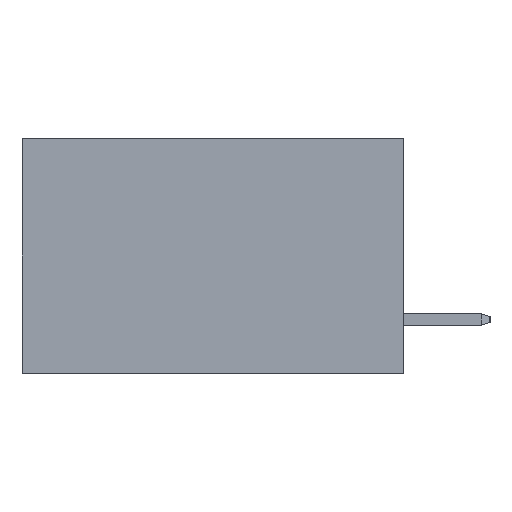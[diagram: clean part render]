
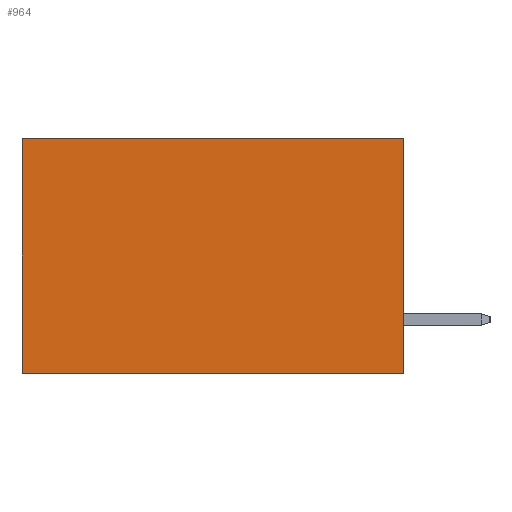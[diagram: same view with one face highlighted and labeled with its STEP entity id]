
A CAD part, left-side view. The second image highlights one B-rep face of the part: STEP entity #964.
In plain terms, the highlighted planar face has unit normal (-1, 0, 0).
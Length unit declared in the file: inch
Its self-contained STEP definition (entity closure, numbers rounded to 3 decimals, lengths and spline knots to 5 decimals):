
#555 = CARTESIAN_POINT ( 'NONE',  ( 0.2875, 0., 0. ) ) ;
#858 = CARTESIAN_POINT ( 'NONE',  ( 0.2875, 0., 0. ) ) ;
#964 = ADVANCED_FACE ( 'NONE', ( #3666 ), #6240, .F. ) ;
#1748 = VERTEX_POINT ( 'NONE', #2897 ) ;
#1966 = ORIENTED_EDGE ( 'NONE', *, *, #9739, .T. ) ;
#2611 = CARTESIAN_POINT ( 'NONE',  ( 0.2875, 0., 0. ) ) ;
#2897 = CARTESIAN_POINT ( 'NONE',  ( 0.2875, 0., -0.37 ) ) ;
#3125 = CARTESIAN_POINT ( 'NONE',  ( 0.2875, 0.6, 0. ) ) ;
#3482 = EDGE_CURVE ( 'NONE', #7500, #5282, #8560, .T. ) ;
#3639 = EDGE_CURVE ( 'NONE', #9727, #1748, #5838, .T. ) ;
#3666 = FACE_OUTER_BOUND ( 'NONE', #4972, .T. ) ;
#3714 = AXIS2_PLACEMENT_3D ( 'NONE', #555, #6927, #9453 ) ;
#4009 = EDGE_CURVE ( 'NONE', #1748, #5282, #5455, .T. ) ;
#4097 = DIRECTION ( 'NONE',  ( 0., 1., 0. ) ) ;
#4133 = CARTESIAN_POINT ( 'NONE',  ( 0.2875, 0., 0. ) ) ;
#4531 = VECTOR ( 'NONE', #7599, 39.37008 ) ;
#4972 = EDGE_LOOP ( 'NONE', ( #5570, #9277, #8629, #1966 ) ) ;
#5282 = VERTEX_POINT ( 'NONE', #7859 ) ;
#5455 = LINE ( 'NONE', #9134, #10159 ) ;
#5570 = ORIENTED_EDGE ( 'NONE', *, *, #3482, .T. ) ;
#5838 = LINE ( 'NONE', #858, #9931 ) ;
#6240 = PLANE ( 'NONE',  #3714 ) ;
#6607 = LINE ( 'NONE', #2611, #8314 ) ;
#6864 = CARTESIAN_POINT ( 'NONE',  ( 0.2875, 0.6, 0. ) ) ;
#6927 = DIRECTION ( 'NONE',  ( 1., 0., 0. ) ) ;
#7500 = VERTEX_POINT ( 'NONE', #3125 ) ;
#7599 = DIRECTION ( 'NONE',  ( 0., 0., -1. ) ) ;
#7859 = CARTESIAN_POINT ( 'NONE',  ( 0.2875, 0.6, -0.37 ) ) ;
#8144 = DIRECTION ( 'NONE',  ( 0., 1., 0. ) ) ;
#8314 = VECTOR ( 'NONE', #8144, 39.37008 ) ;
#8560 = LINE ( 'NONE', #6864, #4531 ) ;
#8629 = ORIENTED_EDGE ( 'NONE', *, *, #3639, .F. ) ;
#9009 = DIRECTION ( 'NONE',  ( 0., 0., -1. ) ) ;
#9134 = CARTESIAN_POINT ( 'NONE',  ( 0.2875, 0., -0.37 ) ) ;
#9277 = ORIENTED_EDGE ( 'NONE', *, *, #4009, .F. ) ;
#9453 = DIRECTION ( 'NONE',  ( 0., 0., -1. ) ) ;
#9727 = VERTEX_POINT ( 'NONE', #4133 ) ;
#9739 = EDGE_CURVE ( 'NONE', #9727, #7500, #6607, .T. ) ;
#9931 = VECTOR ( 'NONE', #9009, 39.37008 ) ;
#10159 = VECTOR ( 'NONE', #4097, 39.37008 ) ;
